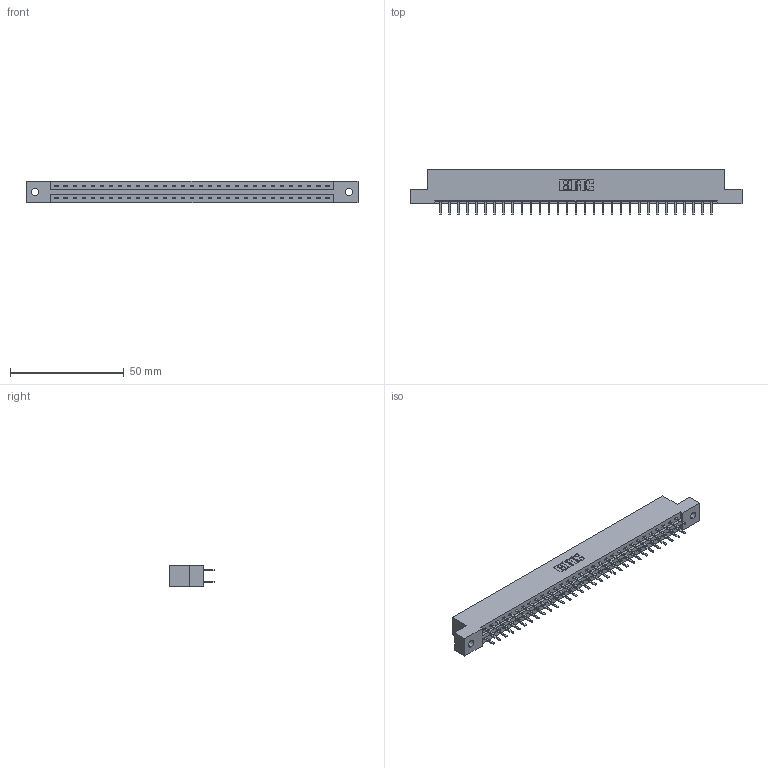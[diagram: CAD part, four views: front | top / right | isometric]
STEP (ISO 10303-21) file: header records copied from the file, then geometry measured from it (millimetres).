
FILE_DESCRIPTION (( 'STEP AP203' ), '1' );
FILE_NAME ('337-062-520-202.STEP', '2019-10-09T21:01:55', ( '' ), ( '' ), 'SwSTEP 2.0', 'SolidWorks 2016', '' );
FILE_SCHEMA (( 'CONFIG_CONTROL_DESIGN' ));
Length unit declared in the file: inch
Products named in the file (3): 345-292-001_345-293-120; 337-062-520-202; 337 Part_Flush Mounting Lugs - 0.128 Dia
Assembly tree (63 placements, depth 2):
  337-062-520-202
    337 Part_Flush Mounting Lugs - 0.128 Dia
    345-292-001_345-293-120  x62
Bounding box: 145.85 x 20.02 x 9.4 mm (x, y, z)
Volume: 15160.1 mm3; surface area: 16681.3 mm2
Topology: 63 solids, 63 shells, 3710 faces, 10789 edges, 7026 vertices
Faces by surface type: plane 2550, cylinder 1160
Entity records: 25575 total; most frequent: CARTESIAN_POINT 4330, ORIENTED_EDGE 4254, DIRECTION 3691, EDGE_CURVE 2127, VECTOR 1995, LINE 1995, VERTEX_POINT 1414, AXIS2_PLACEMENT_3D 848
